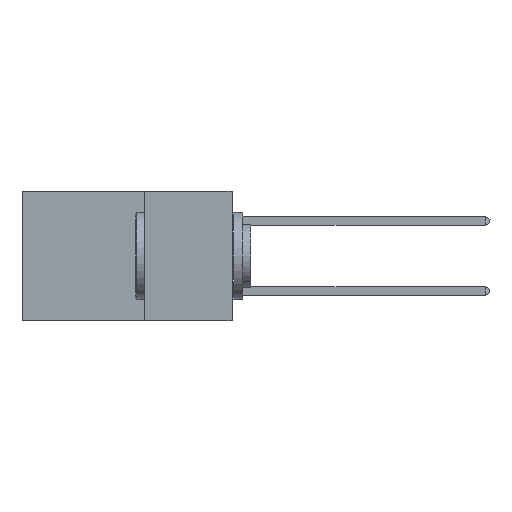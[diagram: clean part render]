
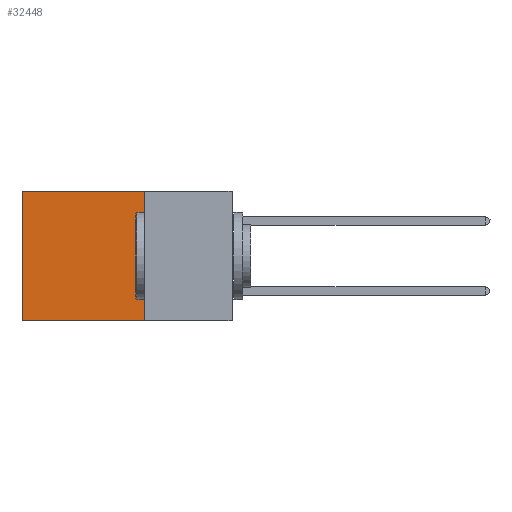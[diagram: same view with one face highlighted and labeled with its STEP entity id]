
A CAD part, left-side view. The second image highlights one B-rep face of the part: STEP entity #32448.
In plain terms, the highlighted planar face has unit normal (-1, 0, 0).
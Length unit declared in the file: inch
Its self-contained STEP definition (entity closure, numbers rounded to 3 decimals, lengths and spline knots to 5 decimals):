
#189 = ORIENTED_EDGE ( 'NONE', *, *, #18484, .T. ) ;
#1585 = AXIS2_PLACEMENT_3D ( 'NONE', #37495, #12609, #18734 ) ;
#3324 = VERTEX_POINT ( 'NONE', #4898 ) ;
#3904 = ORIENTED_EDGE ( 'NONE', *, *, #34127, .T. ) ;
#4493 = DIRECTION ( 'NONE',  ( 0., 1., 0. ) ) ;
#4898 = CARTESIAN_POINT ( 'NONE',  ( 0.2875, 0.6, 0. ) ) ;
#9001 = VECTOR ( 'NONE', #4493, 39.37008 ) ;
#10059 = CARTESIAN_POINT ( 'NONE',  ( 0.2875, 0.6, -0.37 ) ) ;
#10512 = DIRECTION ( 'NONE',  ( 0., 0., -1. ) ) ;
#12446 = VERTEX_POINT ( 'NONE', #10059 ) ;
#12609 = DIRECTION ( 'NONE',  ( 1., 0., 0. ) ) ;
#13183 = VERTEX_POINT ( 'NONE', #18554 ) ;
#13529 = EDGE_CURVE ( 'NONE', #29903, #12446, #18011, .T. ) ;
#13637 = DIRECTION ( 'NONE',  ( 0., 1., 0. ) ) ;
#14740 = VECTOR ( 'NONE', #10512, 39.37008 ) ;
#15035 = ORIENTED_EDGE ( 'NONE', *, *, #13529, .F. ) ;
#15342 = CARTESIAN_POINT ( 'NONE',  ( 0.2875, 0.25, -0.37 ) ) ;
#15643 = PLANE ( 'NONE',  #1585 ) ;
#18011 = LINE ( 'NONE', #15342, #24358 ) ;
#18484 = EDGE_CURVE ( 'NONE', #3324, #12446, #25393, .T. ) ;
#18554 = CARTESIAN_POINT ( 'NONE',  ( 0.2875, 0.25, 0. ) ) ;
#18734 = DIRECTION ( 'NONE',  ( 0., 0., -1. ) ) ;
#19976 = CARTESIAN_POINT ( 'NONE',  ( 0.2875, 0.25, 0. ) ) ;
#24093 = EDGE_CURVE ( 'NONE', #13183, #29903, #36096, .T. ) ;
#24358 = VECTOR ( 'NONE', #13637, 39.37008 ) ;
#25393 = LINE ( 'NONE', #26111, #14740 ) ;
#25475 = CARTESIAN_POINT ( 'NONE',  ( 0.2875, 0.25, -0.37 ) ) ;
#25643 = ORIENTED_EDGE ( 'NONE', *, *, #24093, .F. ) ;
#26111 = CARTESIAN_POINT ( 'NONE',  ( 0.2875, 0.6, 0. ) ) ;
#27105 = LINE ( 'NONE', #19976, #9001 ) ;
#27765 = VECTOR ( 'NONE', #34480, 39.37008 ) ;
#29903 = VERTEX_POINT ( 'NONE', #25475 ) ;
#30801 = EDGE_LOOP ( 'NONE', ( #189, #15035, #25643, #3904 ) ) ;
#32448 = ADVANCED_FACE ( 'NONE', ( #34273 ), #15643, .F. ) ;
#34127 = EDGE_CURVE ( 'NONE', #13183, #3324, #27105, .T. ) ;
#34273 = FACE_OUTER_BOUND ( 'NONE', #30801, .T. ) ;
#34480 = DIRECTION ( 'NONE',  ( 0., 0., -1. ) ) ;
#34722 = CARTESIAN_POINT ( 'NONE',  ( 0.2875, 0.25, 0. ) ) ;
#36096 = LINE ( 'NONE', #34722, #27765 ) ;
#37495 = CARTESIAN_POINT ( 'NONE',  ( 0.2875, 0.25, 0. ) ) ;
